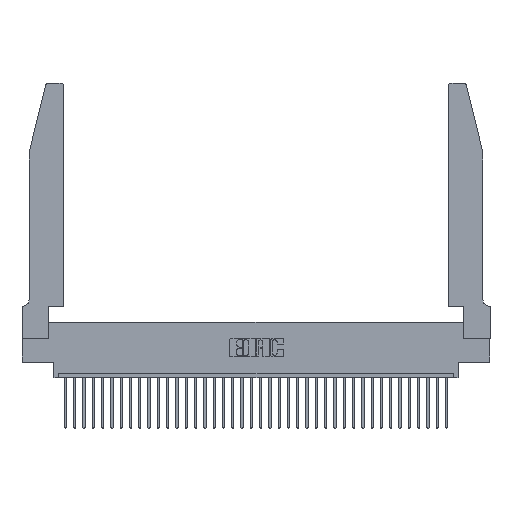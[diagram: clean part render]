
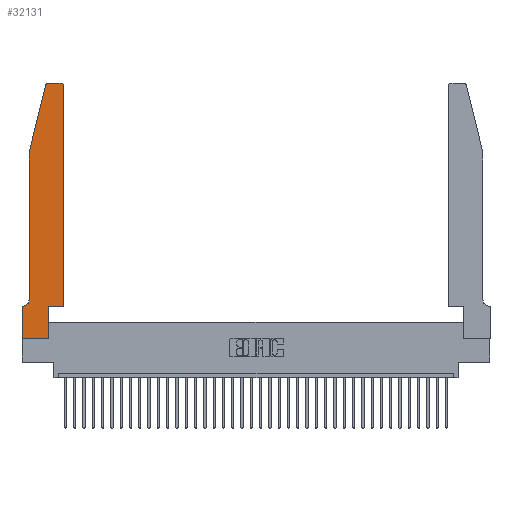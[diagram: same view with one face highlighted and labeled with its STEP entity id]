
A CAD part, top view. The second image highlights one B-rep face of the part: STEP entity #32131.
In plain terms, the highlighted planar face has unit normal (0, 0, 1).
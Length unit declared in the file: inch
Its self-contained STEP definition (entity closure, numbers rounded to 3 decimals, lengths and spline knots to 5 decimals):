
#28 = ORIENTED_EDGE ( 'NONE', *, *, #1350, .T. ) ;
#907 = ORIENTED_EDGE ( 'NONE', *, *, #15880, .T. ) ;
#1305 = VECTOR ( 'NONE', #11672, 39.37008 ) ;
#1350 = EDGE_CURVE ( 'NONE', #25842, #27498, #35412, .T. ) ;
#1476 = CARTESIAN_POINT ( 'NONE',  ( 0.0055, 0.35, 0.37 ) ) ;
#1759 = ORIENTED_EDGE ( 'NONE', *, *, #34003, .T. ) ;
#1976 = DIRECTION ( 'NONE',  ( -1., 0., 0. ) ) ;
#2175 = ORIENTED_EDGE ( 'NONE', *, *, #30728, .T. ) ;
#2200 = LINE ( 'NONE', #14643, #1305 ) ;
#2697 = VECTOR ( 'NONE', #28925, 39.37008 ) ;
#4117 = CIRCLE ( 'NONE', #35885, 0.07 ) ;
#4770 = CARTESIAN_POINT ( 'NONE',  ( 0.0755, 0.42, 0.37 ) ) ;
#4976 = VERTEX_POINT ( 'NONE', #1476 ) ;
#5407 = ORIENTED_EDGE ( 'NONE', *, *, #6090, .T. ) ;
#5523 = DIRECTION ( 'NONE',  ( 0., 0., 1. ) ) ;
#5757 = DIRECTION ( 'NONE',  ( 1., 0., 0. ) ) ;
#5859 = ORIENTED_EDGE ( 'NONE', *, *, #24361, .T. ) ;
#6018 = CARTESIAN_POINT ( 'NONE',  ( 0.2865, 0.35, 0.37 ) ) ;
#6090 = EDGE_CURVE ( 'NONE', #23952, #11293, #14622, .T. ) ;
#6540 = VECTOR ( 'NONE', #32530, 39.37008 ) ;
#7580 = ORIENTED_EDGE ( 'NONE', *, *, #33773, .T. ) ;
#7801 = VERTEX_POINT ( 'NONE', #35935 ) ;
#8091 = EDGE_CURVE ( 'NONE', #10081, #26849, #21524, .T. ) ;
#8178 = DIRECTION ( 'NONE',  ( 0., 0., 1. ) ) ;
#8441 = VERTEX_POINT ( 'NONE', #23216 ) ;
#8955 = CARTESIAN_POINT ( 'NONE',  ( 0.0755, 2., 0.37 ) ) ;
#9407 = VECTOR ( 'NONE', #35974, 39.37008 ) ;
#10014 = ORIENTED_EDGE ( 'NONE', *, *, #8091, .T. ) ;
#10081 = VERTEX_POINT ( 'NONE', #35859 ) ;
#10242 = DIRECTION ( 'NONE',  ( 1., 0., 0. ) ) ;
#10586 = CARTESIAN_POINT ( 'NONE',  ( 0.2865, 0.35, 0.37 ) ) ;
#10955 = PLANE ( 'NONE',  #22065 ) ;
#11062 = DIRECTION ( 'NONE',  ( -1., 0., 0. ) ) ;
#11293 = VERTEX_POINT ( 'NONE', #26247 ) ;
#11672 = DIRECTION ( 'NONE',  ( -0.239, -0.971, 0. ) ) ;
#11926 = ORIENTED_EDGE ( 'NONE', *, *, #26536, .T. ) ;
#12152 = CARTESIAN_POINT ( 'NONE',  ( 0.0755, 2., 0.37 ) ) ;
#12617 = VECTOR ( 'NONE', #1976, 39.37008 ) ;
#13949 = LINE ( 'NONE', #12152, #32881 ) ;
#14616 = EDGE_CURVE ( 'NONE', #4976, #23952, #30689, .T. ) ;
#14622 = LINE ( 'NONE', #35410, #2697 ) ;
#14643 = CARTESIAN_POINT ( 'NONE',  ( 0.0755, 2., 0.37 ) ) ;
#14728 = LINE ( 'NONE', #10586, #9407 ) ;
#15880 = EDGE_CURVE ( 'NONE', #27498, #27133, #34138, .T. ) ;
#16788 = LINE ( 'NONE', #18609, #22061 ) ;
#18609 = CARTESIAN_POINT ( 'NONE',  ( 0., 0., 0.37 ) ) ;
#19083 = AXIS2_PLACEMENT_3D ( 'NONE', #27883, #5523, #19553 ) ;
#19553 = DIRECTION ( 'NONE',  ( 1., 0., 0. ) ) ;
#20404 = VECTOR ( 'NONE', #29750, 39.37008 ) ;
#20626 = DIRECTION ( 'NONE',  ( 0., -1., 0. ) ) ;
#21338 = VECTOR ( 'NONE', #21744, 39.37008 ) ;
#21524 = LINE ( 'NONE', #27295, #6540 ) ;
#21744 = DIRECTION ( 'NONE',  ( 0., 1., 0. ) ) ;
#21773 = CARTESIAN_POINT ( 'NONE',  ( 0.4505, 0.35, 0.37 ) ) ;
#22061 = VECTOR ( 'NONE', #10242, 39.37008 ) ;
#22065 = AXIS2_PLACEMENT_3D ( 'NONE', #30791, #22271, #5757 ) ;
#22188 = EDGE_CURVE ( 'NONE', #7801, #25842, #14728, .T. ) ;
#22255 = ORIENTED_EDGE ( 'NONE', *, *, #25951, .T. ) ;
#22271 = DIRECTION ( 'NONE',  ( 0., 0., 1. ) ) ;
#23216 = CARTESIAN_POINT ( 'NONE',  ( 0.25487, 2.72718, 0.37 ) ) ;
#23818 = AXIS2_PLACEMENT_3D ( 'NONE', #27729, #8178, #27954 ) ;
#23952 = VERTEX_POINT ( 'NONE', #30921 ) ;
#24361 = EDGE_CURVE ( 'NONE', #26849, #8441, #31573, .T. ) ;
#25271 = CARTESIAN_POINT ( 'NONE',  ( 0.0055, 0.42, 0.37 ) ) ;
#25842 = VERTEX_POINT ( 'NONE', #6018 ) ;
#25951 = EDGE_CURVE ( 'NONE', #27133, #10081, #26225, .T. ) ;
#26206 = FACE_OUTER_BOUND ( 'NONE', #31578, .T. ) ;
#26225 = CIRCLE ( 'NONE', #19083, 0.03 ) ;
#26247 = CARTESIAN_POINT ( 'NONE',  ( 0., 0., 0.37 ) ) ;
#26536 = EDGE_CURVE ( 'NONE', #35913, #4976, #4117, .T. ) ;
#26849 = VERTEX_POINT ( 'NONE', #31868 ) ;
#27133 = VERTEX_POINT ( 'NONE', #35819 ) ;
#27289 = CARTESIAN_POINT ( 'NONE',  ( 0.0755, 0.35, 0.37 ) ) ;
#27295 = CARTESIAN_POINT ( 'NONE',  ( 0.2605, 2.75, 0.37 ) ) ;
#27415 = ORIENTED_EDGE ( 'NONE', *, *, #22188, .T. ) ;
#27498 = VERTEX_POINT ( 'NONE', #21773 ) ;
#27729 = CARTESIAN_POINT ( 'NONE',  ( 0.284, 2.72, 0.37 ) ) ;
#27883 = CARTESIAN_POINT ( 'NONE',  ( 0.4205, 2.72, 0.37 ) ) ;
#27954 = DIRECTION ( 'NONE',  ( 1., 0., 0. ) ) ;
#28925 = DIRECTION ( 'NONE',  ( 0., -1., 0. ) ) ;
#29750 = DIRECTION ( 'NONE',  ( 1., 0., 0. ) ) ;
#30370 = CARTESIAN_POINT ( 'NONE',  ( 0.4505, 0.35, 0.37 ) ) ;
#30689 = LINE ( 'NONE', #27289, #12617 ) ;
#30728 = EDGE_CURVE ( 'NONE', #34092, #35913, #13949, .T. ) ;
#30791 = CARTESIAN_POINT ( 'NONE',  ( 0., 0.35, 0.37 ) ) ;
#30921 = CARTESIAN_POINT ( 'NONE',  ( 0., 0.35, 0.37 ) ) ;
#31573 = CIRCLE ( 'NONE', #23818, 0.03 ) ;
#31578 = EDGE_LOOP ( 'NONE', ( #10014, #5859, #1759, #2175, #11926, #31990, #5407, #7580, #27415, #28, #907, #22255 ) ) ;
#31868 = CARTESIAN_POINT ( 'NONE',  ( 0.284, 2.75, 0.37 ) ) ;
#31990 = ORIENTED_EDGE ( 'NONE', *, *, #14616, .T. ) ;
#32131 = ADVANCED_FACE ( 'NONE', ( #26206 ), #10955, .T. ) ;
#32200 = CARTESIAN_POINT ( 'NONE',  ( 0.4505, 0.35, 0.37 ) ) ;
#32530 = DIRECTION ( 'NONE',  ( -1., 0., 0. ) ) ;
#32881 = VECTOR ( 'NONE', #20626, 39.37008 ) ;
#33773 = EDGE_CURVE ( 'NONE', #11293, #7801, #16788, .T. ) ;
#33843 = DIRECTION ( 'NONE',  ( 0., 0., -1. ) ) ;
#34003 = EDGE_CURVE ( 'NONE', #8441, #34092, #2200, .T. ) ;
#34092 = VERTEX_POINT ( 'NONE', #8955 ) ;
#34138 = LINE ( 'NONE', #30370, #21338 ) ;
#35410 = CARTESIAN_POINT ( 'NONE',  ( 0., 0., 0.37 ) ) ;
#35412 = LINE ( 'NONE', #32200, #20404 ) ;
#35819 = CARTESIAN_POINT ( 'NONE',  ( 0.4505, 2.72, 0.37 ) ) ;
#35859 = CARTESIAN_POINT ( 'NONE',  ( 0.4205, 2.75, 0.37 ) ) ;
#35885 = AXIS2_PLACEMENT_3D ( 'NONE', #25271, #33843, #11062 ) ;
#35913 = VERTEX_POINT ( 'NONE', #4770 ) ;
#35935 = CARTESIAN_POINT ( 'NONE',  ( 0.2865, 0., 0.37 ) ) ;
#35974 = DIRECTION ( 'NONE',  ( 0., 1., 0. ) ) ;
